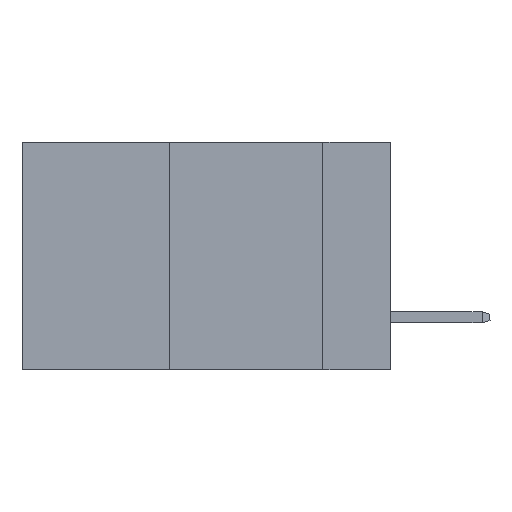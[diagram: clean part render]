
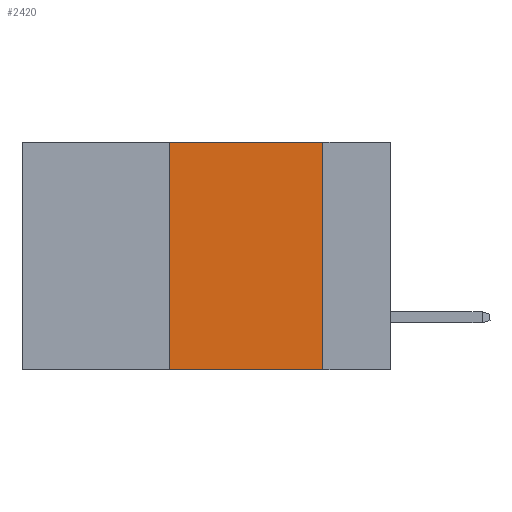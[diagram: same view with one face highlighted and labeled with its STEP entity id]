
A CAD part, left-side view. The second image highlights one B-rep face of the part: STEP entity #2420.
In plain terms, the highlighted planar face has unit normal (-1, 0, 0).
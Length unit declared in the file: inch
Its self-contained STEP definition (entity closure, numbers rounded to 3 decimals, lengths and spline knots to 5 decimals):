
#830 = VERTEX_POINT ( 'NONE', #7460 ) ;
#971 = DIRECTION ( 'NONE',  ( 1., 0., 0. ) ) ;
#1017 = LINE ( 'NONE', #3425, #9782 ) ;
#2018 = AXIS2_PLACEMENT_3D ( 'NONE', #2266, #971, #13653 ) ;
#2132 = VERTEX_POINT ( 'NONE', #2215 ) ;
#2215 = CARTESIAN_POINT ( 'NONE',  ( 0., 0.36, 0. ) ) ;
#2266 = CARTESIAN_POINT ( 'NONE',  ( 0., 0.6, 0. ) ) ;
#2420 = ADVANCED_FACE ( 'NONE', ( #6865 ), #6395, .F. ) ;
#3425 = CARTESIAN_POINT ( 'NONE',  ( 0., 0.6, -0.37 ) ) ;
#3769 = CARTESIAN_POINT ( 'NONE',  ( 0., 0.36, 0. ) ) ;
#4080 = VECTOR ( 'NONE', #9175, 39.37008 ) ;
#4487 = LINE ( 'NONE', #5378, #9888 ) ;
#4592 = VECTOR ( 'NONE', #10311, 39.37008 ) ;
#4800 = EDGE_LOOP ( 'NONE', ( #6173, #5187, #5295, #4828 ) ) ;
#4828 = ORIENTED_EDGE ( 'NONE', *, *, #5083, .T. ) ;
#5083 = EDGE_CURVE ( 'NONE', #7987, #7884, #1017, .T. ) ;
#5187 = ORIENTED_EDGE ( 'NONE', *, *, #8479, .F. ) ;
#5295 = ORIENTED_EDGE ( 'NONE', *, *, #7234, .F. ) ;
#5306 = CARTESIAN_POINT ( 'NONE',  ( 0., 0.36, -0.37 ) ) ;
#5378 = CARTESIAN_POINT ( 'NONE',  ( 0., 0.11, 0. ) ) ;
#6173 = ORIENTED_EDGE ( 'NONE', *, *, #11344, .F. ) ;
#6232 = CARTESIAN_POINT ( 'NONE',  ( 0., 0.11, -0.37 ) ) ;
#6395 = PLANE ( 'NONE',  #2018 ) ;
#6702 = DIRECTION ( 'NONE',  ( 0., -1., 0. ) ) ;
#6865 = FACE_OUTER_BOUND ( 'NONE', #4800, .T. ) ;
#7234 = EDGE_CURVE ( 'NONE', #7987, #2132, #9174, .T. ) ;
#7460 = CARTESIAN_POINT ( 'NONE',  ( 0., 0.11, 0. ) ) ;
#7462 = LINE ( 'NONE', #8201, #4592 ) ;
#7884 = VERTEX_POINT ( 'NONE', #6232 ) ;
#7987 = VERTEX_POINT ( 'NONE', #5306 ) ;
#8201 = CARTESIAN_POINT ( 'NONE',  ( 0., 0.6, 0. ) ) ;
#8479 = EDGE_CURVE ( 'NONE', #2132, #830, #7462, .T. ) ;
#9174 = LINE ( 'NONE', #3769, #4080 ) ;
#9175 = DIRECTION ( 'NONE',  ( 0., 0., 1. ) ) ;
#9782 = VECTOR ( 'NONE', #6702, 39.37008 ) ;
#9888 = VECTOR ( 'NONE', #13545, 39.37008 ) ;
#10311 = DIRECTION ( 'NONE',  ( 0., -1., 0. ) ) ;
#11344 = EDGE_CURVE ( 'NONE', #830, #7884, #4487, .T. ) ;
#13545 = DIRECTION ( 'NONE',  ( 0., 0., -1. ) ) ;
#13653 = DIRECTION ( 'NONE',  ( 0., 0., -1. ) ) ;
